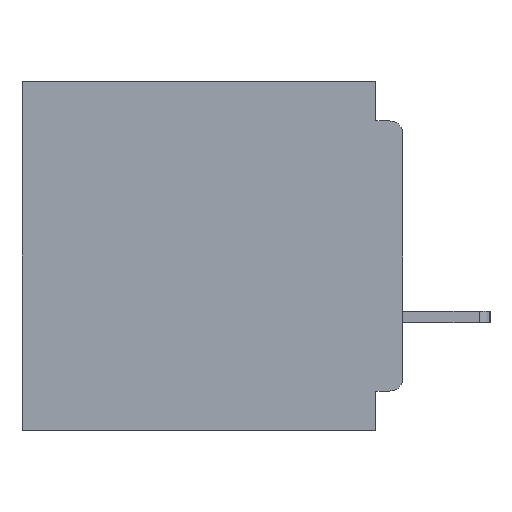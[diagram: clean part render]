
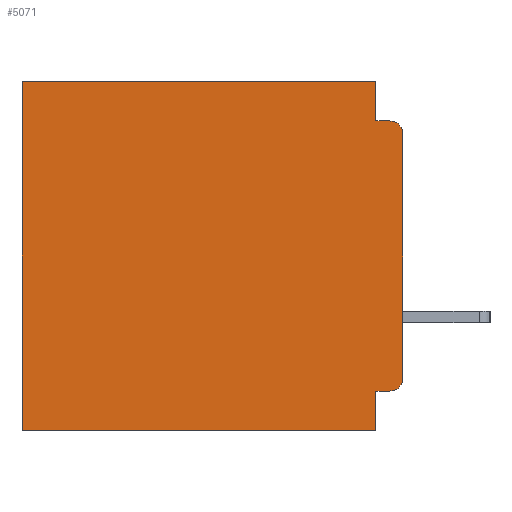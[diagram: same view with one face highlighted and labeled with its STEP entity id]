
A CAD part, left-side view. The second image highlights one B-rep face of the part: STEP entity #5071.
In plain terms, the highlighted planar face has unit normal (-1, 0, 0).
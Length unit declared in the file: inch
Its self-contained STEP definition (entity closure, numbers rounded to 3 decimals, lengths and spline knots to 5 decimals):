
#1078 = CARTESIAN_POINT ( 'NONE',  ( 0.3, 0.437, -0.4 ) ) ;
#1782 = VECTOR ( 'NONE', #30357, 39.37008 ) ;
#2450 = CARTESIAN_POINT ( 'NONE',  ( 0.3, 0., -0.045 ) ) ;
#2712 = CARTESIAN_POINT ( 'NONE',  ( 0.3, 0.437, 0. ) ) ;
#3110 = CIRCLE ( 'NONE', #17929, 0.015 ) ;
#3763 = ORIENTED_EDGE ( 'NONE', *, *, #26143, .F. ) ;
#3782 = DIRECTION ( 'NONE',  ( 0., 0., -1. ) ) ;
#3827 = DIRECTION ( 'NONE',  ( 1., 0., 0. ) ) ;
#4456 = ORIENTED_EDGE ( 'NONE', *, *, #17731, .T. ) ;
#5071 = ADVANCED_FACE ( 'NONE', ( #43474 ), #11600, .F. ) ;
#5567 = ORIENTED_EDGE ( 'NONE', *, *, #31655, .F. ) ;
#5678 = CARTESIAN_POINT ( 'NONE',  ( 0.3, 0.031, 0. ) ) ;
#6341 = VECTOR ( 'NONE', #14319, 39.37008 ) ;
#6673 = CARTESIAN_POINT ( 'NONE',  ( 0.3, 0.031, 0. ) ) ;
#7458 = LINE ( 'NONE', #24617, #6341 ) ;
#8257 = LINE ( 'NONE', #11464, #18582 ) ;
#9583 = VERTEX_POINT ( 'NONE', #25364 ) ;
#9866 = EDGE_CURVE ( 'NONE', #32297, #29796, #44635, .T. ) ;
#10204 = CARTESIAN_POINT ( 'NONE',  ( 0.3, 0., -0.4 ) ) ;
#10555 = CARTESIAN_POINT ( 'NONE',  ( 0.3, 0., -0.34 ) ) ;
#11464 = CARTESIAN_POINT ( 'NONE',  ( 0.3, 0.031, -0.4 ) ) ;
#11600 = PLANE ( 'NONE',  #14483 ) ;
#11855 = VERTEX_POINT ( 'NONE', #6673 ) ;
#13393 = DIRECTION ( 'NONE',  ( -1., 0., 0. ) ) ;
#14103 = CARTESIAN_POINT ( 'NONE',  ( 0.3, 0.031, -0.355 ) ) ;
#14319 = DIRECTION ( 'NONE',  ( 0., 1., 0. ) ) ;
#14483 = AXIS2_PLACEMENT_3D ( 'NONE', #10204, #3827, #3782 ) ;
#14869 = DIRECTION ( 'NONE',  ( 0., 1., 0. ) ) ;
#15261 = DIRECTION ( 'NONE',  ( 0., 0., -1. ) ) ;
#15589 = DIRECTION ( 'NONE',  ( 0., 0., -1. ) ) ;
#17415 = ORIENTED_EDGE ( 'NONE', *, *, #39871, .T. ) ;
#17731 = EDGE_CURVE ( 'NONE', #9583, #35038, #3110, .T. ) ;
#17929 = AXIS2_PLACEMENT_3D ( 'NONE', #34216, #13393, #37695 ) ;
#17983 = EDGE_CURVE ( 'NONE', #41243, #39980, #36377, .T. ) ;
#18094 = CARTESIAN_POINT ( 'NONE',  ( 0.3, 0.031, -0.4 ) ) ;
#18582 = VECTOR ( 'NONE', #25236, 39.37008 ) ;
#18600 = CARTESIAN_POINT ( 'NONE',  ( 0.3, 0., -0.06 ) ) ;
#19117 = VECTOR ( 'NONE', #43981, 39.37008 ) ;
#19832 = CARTESIAN_POINT ( 'NONE',  ( 0.3, 0., -0.355 ) ) ;
#20790 = CARTESIAN_POINT ( 'NONE',  ( 0.3, 0.015, -0.06 ) ) ;
#20890 = VECTOR ( 'NONE', #15261, 39.37008 ) ;
#21129 = LINE ( 'NONE', #23141, #37509 ) ;
#23141 = CARTESIAN_POINT ( 'NONE',  ( 0.3, 0.437, -0.4 ) ) ;
#24083 = ORIENTED_EDGE ( 'NONE', *, *, #39798, .F. ) ;
#24289 = DIRECTION ( 'NONE',  ( 0., 0., -1. ) ) ;
#24469 = DIRECTION ( 'NONE',  ( 0., 0., -1. ) ) ;
#24617 = CARTESIAN_POINT ( 'NONE',  ( 0.3, 0., 0. ) ) ;
#25236 = DIRECTION ( 'NONE',  ( 0., 0., -1. ) ) ;
#25262 = ORIENTED_EDGE ( 'NONE', *, *, #17983, .F. ) ;
#25364 = CARTESIAN_POINT ( 'NONE',  ( 0.3, 0.015, -0.355 ) ) ;
#26143 = EDGE_CURVE ( 'NONE', #26146, #35038, #39406, .T. ) ;
#26146 = VERTEX_POINT ( 'NONE', #18600 ) ;
#26988 = EDGE_CURVE ( 'NONE', #26146, #29796, #39325, .T. ) ;
#27658 = VERTEX_POINT ( 'NONE', #14103 ) ;
#27734 = EDGE_LOOP ( 'NONE', ( #3763, #42877, #37033, #24083, #17415, #31814, #25262, #41776, #5567, #4456 ) ) ;
#28007 = VERTEX_POINT ( 'NONE', #2712 ) ;
#28103 = VECTOR ( 'NONE', #24469, 39.37008 ) ;
#28659 = CARTESIAN_POINT ( 'NONE',  ( 0.3, 0., -0.4 ) ) ;
#29796 = VERTEX_POINT ( 'NONE', #43849 ) ;
#30357 = DIRECTION ( 'NONE',  ( 0., -1., 0. ) ) ;
#30423 = AXIS2_PLACEMENT_3D ( 'NONE', #20790, #44903, #24289 ) ;
#31655 = EDGE_CURVE ( 'NONE', #9583, #27658, #38709, .T. ) ;
#31814 = ORIENTED_EDGE ( 'NONE', *, *, #32892, .T. ) ;
#32297 = VERTEX_POINT ( 'NONE', #38068 ) ;
#32892 = EDGE_CURVE ( 'NONE', #28007, #39980, #21129, .T. ) ;
#34216 = CARTESIAN_POINT ( 'NONE',  ( 0.3, 0.015, -0.34 ) ) ;
#35038 = VERTEX_POINT ( 'NONE', #10555 ) ;
#36330 = LINE ( 'NONE', #5678, #28103 ) ;
#36377 = LINE ( 'NONE', #28659, #44298 ) ;
#37033 = ORIENTED_EDGE ( 'NONE', *, *, #9866, .F. ) ;
#37509 = VECTOR ( 'NONE', #15589, 39.37008 ) ;
#37516 = EDGE_CURVE ( 'NONE', #27658, #41243, #8257, .T. ) ;
#37695 = DIRECTION ( 'NONE',  ( 0., 0., -1. ) ) ;
#38068 = CARTESIAN_POINT ( 'NONE',  ( 0.3, 0.031, -0.045 ) ) ;
#38709 = LINE ( 'NONE', #19832, #19117 ) ;
#39325 = CIRCLE ( 'NONE', #30423, 0.015 ) ;
#39406 = LINE ( 'NONE', #39564, #20890 ) ;
#39564 = CARTESIAN_POINT ( 'NONE',  ( 0.3, 0., -0.4 ) ) ;
#39798 = EDGE_CURVE ( 'NONE', #11855, #32297, #36330, .T. ) ;
#39871 = EDGE_CURVE ( 'NONE', #11855, #28007, #7458, .T. ) ;
#39980 = VERTEX_POINT ( 'NONE', #1078 ) ;
#41243 = VERTEX_POINT ( 'NONE', #18094 ) ;
#41776 = ORIENTED_EDGE ( 'NONE', *, *, #37516, .F. ) ;
#42877 = ORIENTED_EDGE ( 'NONE', *, *, #26988, .T. ) ;
#43474 = FACE_OUTER_BOUND ( 'NONE', #27734, .T. ) ;
#43849 = CARTESIAN_POINT ( 'NONE',  ( 0.3, 0.015, -0.045 ) ) ;
#43981 = DIRECTION ( 'NONE',  ( 0., 1., 0. ) ) ;
#44298 = VECTOR ( 'NONE', #14869, 39.37008 ) ;
#44635 = LINE ( 'NONE', #2450, #1782 ) ;
#44903 = DIRECTION ( 'NONE',  ( -1., 0., 0. ) ) ;
